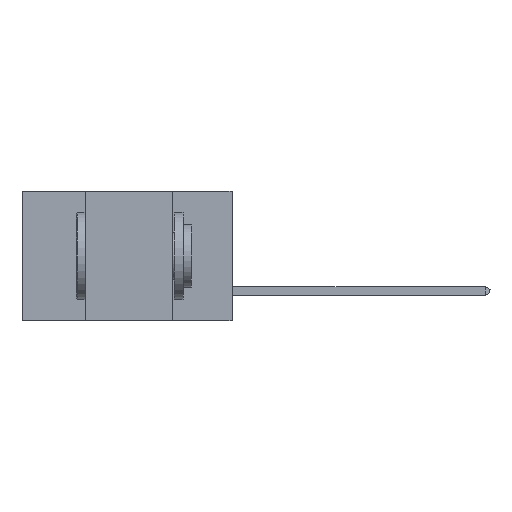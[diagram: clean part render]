
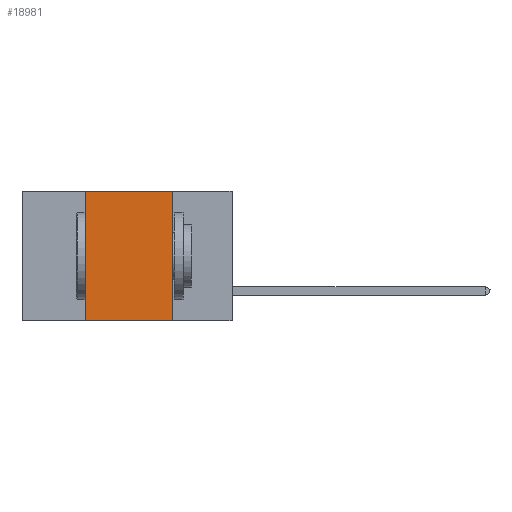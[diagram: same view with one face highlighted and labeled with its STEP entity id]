
A CAD part, left-side view. The second image highlights one B-rep face of the part: STEP entity #18981.
In plain terms, the highlighted planar face has unit normal (-1, 0, 0).
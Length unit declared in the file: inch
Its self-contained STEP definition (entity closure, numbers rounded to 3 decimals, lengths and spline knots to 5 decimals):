
#363 = VECTOR ( 'NONE', #24357, 39.37008 ) ;
#1398 = DIRECTION ( 'NONE',  ( 0., 0., -1. ) ) ;
#1707 = PLANE ( 'NONE',  #19788 ) ;
#4694 = CARTESIAN_POINT ( 'NONE',  ( 0., 0.17, 0. ) ) ;
#5710 = CARTESIAN_POINT ( 'NONE',  ( 0., 0.17, -0.37 ) ) ;
#5814 = VERTEX_POINT ( 'NONE', #8336 ) ;
#8336 = CARTESIAN_POINT ( 'NONE',  ( 0., 0.42, 0. ) ) ;
#10193 = LINE ( 'NONE', #34237, #363 ) ;
#11033 = VECTOR ( 'NONE', #12000, 39.37008 ) ;
#11357 = EDGE_LOOP ( 'NONE', ( #24554, #18513, #30753, #42736 ) ) ;
#12000 = DIRECTION ( 'NONE',  ( 0., 0., -1. ) ) ;
#13633 = DIRECTION ( 'NONE',  ( 0., -1., 0. ) ) ;
#14563 = VERTEX_POINT ( 'NONE', #28033 ) ;
#16464 = EDGE_CURVE ( 'NONE', #14563, #30952, #10193, .T. ) ;
#17675 = LINE ( 'NONE', #4694, #11033 ) ;
#18170 = LINE ( 'NONE', #40710, #32640 ) ;
#18513 = ORIENTED_EDGE ( 'NONE', *, *, #25915, .F. ) ;
#18981 = ADVANCED_FACE ( 'NONE', ( #40858 ), #1707, .F. ) ;
#19788 = AXIS2_PLACEMENT_3D ( 'NONE', #41151, #21702, #1398 ) ;
#21702 = DIRECTION ( 'NONE',  ( 1., 0., 0. ) ) ;
#22110 = LINE ( 'NONE', #26496, #33936 ) ;
#24357 = DIRECTION ( 'NONE',  ( 0., -1., 0. ) ) ;
#24554 = ORIENTED_EDGE ( 'NONE', *, *, #39502, .F. ) ;
#25915 = EDGE_CURVE ( 'NONE', #5814, #31574, #22110, .T. ) ;
#26496 = CARTESIAN_POINT ( 'NONE',  ( 0., 0.6, 0. ) ) ;
#28033 = CARTESIAN_POINT ( 'NONE',  ( 0., 0.42, -0.37 ) ) ;
#30657 = EDGE_CURVE ( 'NONE', #14563, #5814, #18170, .T. ) ;
#30753 = ORIENTED_EDGE ( 'NONE', *, *, #30657, .F. ) ;
#30952 = VERTEX_POINT ( 'NONE', #5710 ) ;
#31574 = VERTEX_POINT ( 'NONE', #37951 ) ;
#32640 = VECTOR ( 'NONE', #40989, 39.37008 ) ;
#33936 = VECTOR ( 'NONE', #13633, 39.37008 ) ;
#34237 = CARTESIAN_POINT ( 'NONE',  ( 0., 0.6, -0.37 ) ) ;
#37951 = CARTESIAN_POINT ( 'NONE',  ( 0., 0.17, 0. ) ) ;
#39502 = EDGE_CURVE ( 'NONE', #31574, #30952, #17675, .T. ) ;
#40710 = CARTESIAN_POINT ( 'NONE',  ( 0., 0.42, 0. ) ) ;
#40858 = FACE_OUTER_BOUND ( 'NONE', #11357, .T. ) ;
#40989 = DIRECTION ( 'NONE',  ( 0., 0., 1. ) ) ;
#41151 = CARTESIAN_POINT ( 'NONE',  ( 0., 0.6, 0. ) ) ;
#42736 = ORIENTED_EDGE ( 'NONE', *, *, #16464, .T. ) ;
